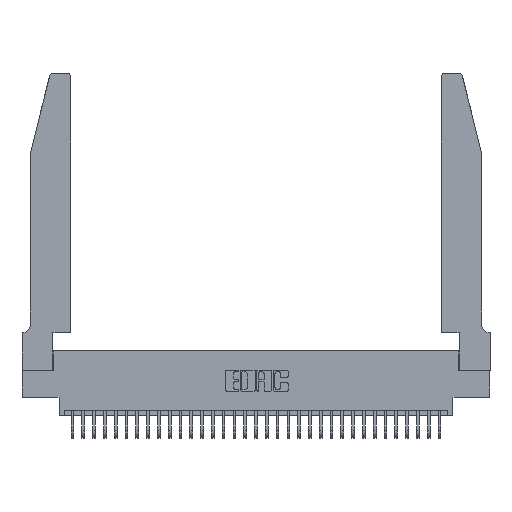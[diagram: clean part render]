
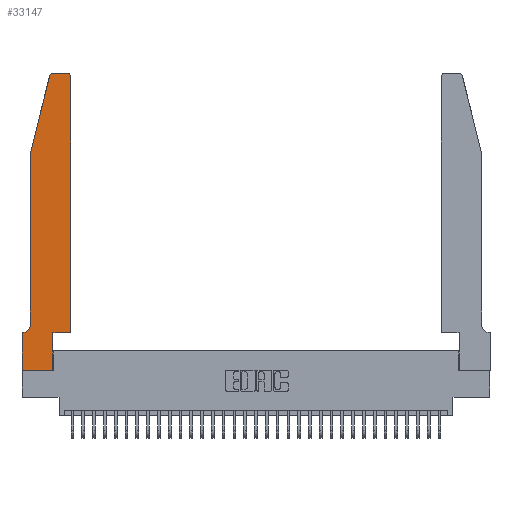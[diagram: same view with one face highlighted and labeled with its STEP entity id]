
A CAD part, top view. The second image highlights one B-rep face of the part: STEP entity #33147.
In plain terms, the highlighted planar face has unit normal (0, 0, 1).
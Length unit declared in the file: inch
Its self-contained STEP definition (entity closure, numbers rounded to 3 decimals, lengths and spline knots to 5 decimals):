
#81 = VECTOR ( 'NONE', #19132, 39.37008 ) ;
#641 = CARTESIAN_POINT ( 'NONE',  ( 0.2865, 0.35, 0.37 ) ) ;
#921 = LINE ( 'NONE', #16429, #81 ) ;
#1046 = LINE ( 'NONE', #18296, #5297 ) ;
#1325 = EDGE_CURVE ( 'NONE', #33380, #15692, #2340, .T. ) ;
#1551 = AXIS2_PLACEMENT_3D ( 'NONE', #29426, #2204, #21242 ) ;
#2133 = LINE ( 'NONE', #12270, #30064 ) ;
#2204 = DIRECTION ( 'NONE',  ( 0., 0., 1. ) ) ;
#2340 = CIRCLE ( 'NONE', #6354, 0.07 ) ;
#2687 = EDGE_LOOP ( 'NONE', ( #6096, #9109, #33235, #9890, #5475, #23231, #8841, #26085, #34514, #3562, #22490, #9394 ) ) ;
#3004 = EDGE_CURVE ( 'NONE', #22376, #18172, #30586, .T. ) ;
#3489 = CARTESIAN_POINT ( 'NONE',  ( 0.25487, 2.72718, 0.37 ) ) ;
#3562 = ORIENTED_EDGE ( 'NONE', *, *, #34745, .T. ) ;
#3617 = EDGE_CURVE ( 'NONE', #4732, #15145, #4727, .T. ) ;
#4388 = LINE ( 'NONE', #11160, #28938 ) ;
#4727 = LINE ( 'NONE', #26970, #11080 ) ;
#4732 = VERTEX_POINT ( 'NONE', #11451 ) ;
#5297 = VECTOR ( 'NONE', #26371, 39.37008 ) ;
#5475 = ORIENTED_EDGE ( 'NONE', *, *, #1325, .T. ) ;
#5584 = CARTESIAN_POINT ( 'NONE',  ( 0., 0., 0.37 ) ) ;
#6096 = ORIENTED_EDGE ( 'NONE', *, *, #33855, .T. ) ;
#6232 = CARTESIAN_POINT ( 'NONE',  ( 0.4505, 0.35, 0.37 ) ) ;
#6354 = AXIS2_PLACEMENT_3D ( 'NONE', #14543, #17375, #22728 ) ;
#7540 = CIRCLE ( 'NONE', #28967, 0.03 ) ;
#8121 = EDGE_CURVE ( 'NONE', #15692, #24479, #921, .T. ) ;
#8638 = VECTOR ( 'NONE', #23850, 39.37008 ) ;
#8841 = ORIENTED_EDGE ( 'NONE', *, *, #15777, .T. ) ;
#9016 = DIRECTION ( 'NONE',  ( 0., 0., 1. ) ) ;
#9109 = ORIENTED_EDGE ( 'NONE', *, *, #32810, .T. ) ;
#9224 = CARTESIAN_POINT ( 'NONE',  ( 0.4205, 2.72, 0.37 ) ) ;
#9394 = ORIENTED_EDGE ( 'NONE', *, *, #19500, .T. ) ;
#9439 = VERTEX_POINT ( 'NONE', #29065 ) ;
#9520 = LINE ( 'NONE', #29454, #8638 ) ;
#9890 = ORIENTED_EDGE ( 'NONE', *, *, #21620, .T. ) ;
#10090 = CARTESIAN_POINT ( 'NONE',  ( 0.4505, 2.72, 0.37 ) ) ;
#11080 = VECTOR ( 'NONE', #19087, 39.37008 ) ;
#11160 = CARTESIAN_POINT ( 'NONE',  ( 0.0755, 2., 0.37 ) ) ;
#11451 = CARTESIAN_POINT ( 'NONE',  ( 0., 0., 0.37 ) ) ;
#11564 = VECTOR ( 'NONE', #30219, 39.37008 ) ;
#11575 = DIRECTION ( 'NONE',  ( 0., 1., 0. ) ) ;
#11954 = DIRECTION ( 'NONE',  ( 0., 0., 1. ) ) ;
#12270 = CARTESIAN_POINT ( 'NONE',  ( 0.4505, 0.35, 0.37 ) ) ;
#13005 = VERTEX_POINT ( 'NONE', #14455 ) ;
#13828 = CARTESIAN_POINT ( 'NONE',  ( 0.4205, 2.75, 0.37 ) ) ;
#14339 = DIRECTION ( 'NONE',  ( 1., 0., 0. ) ) ;
#14455 = CARTESIAN_POINT ( 'NONE',  ( 0.284, 2.75, 0.37 ) ) ;
#14543 = CARTESIAN_POINT ( 'NONE',  ( 0.0055, 0.42, 0.37 ) ) ;
#14791 = DIRECTION ( 'NONE',  ( 1., 0., 0. ) ) ;
#14827 = CARTESIAN_POINT ( 'NONE',  ( 0.284, 2.72, 0.37 ) ) ;
#15145 = VERTEX_POINT ( 'NONE', #25852 ) ;
#15692 = VERTEX_POINT ( 'NONE', #34358 ) ;
#15777 = EDGE_CURVE ( 'NONE', #24479, #4732, #33645, .T. ) ;
#16429 = CARTESIAN_POINT ( 'NONE',  ( 0.0755, 0.35, 0.37 ) ) ;
#17375 = DIRECTION ( 'NONE',  ( 0., 0., -1. ) ) ;
#17505 = CARTESIAN_POINT ( 'NONE',  ( 0., 0.35, 0.37 ) ) ;
#18055 = LINE ( 'NONE', #641, #28146 ) ;
#18172 = VERTEX_POINT ( 'NONE', #27603 ) ;
#18296 = CARTESIAN_POINT ( 'NONE',  ( 0.2605, 2.75, 0.37 ) ) ;
#19087 = DIRECTION ( 'NONE',  ( 1., 0., 0. ) ) ;
#19132 = DIRECTION ( 'NONE',  ( -1., 0., 0. ) ) ;
#19500 = EDGE_CURVE ( 'NONE', #30565, #33425, #7540, .T. ) ;
#20156 = FACE_OUTER_BOUND ( 'NONE', #2687, .T. ) ;
#21242 = DIRECTION ( 'NONE',  ( 1., 0., 0. ) ) ;
#21620 = EDGE_CURVE ( 'NONE', #18172, #33380, #4388, .T. ) ;
#22376 = VERTEX_POINT ( 'NONE', #3489 ) ;
#22490 = ORIENTED_EDGE ( 'NONE', *, *, #23319, .T. ) ;
#22609 = VECTOR ( 'NONE', #30679, 39.37008 ) ;
#22728 = DIRECTION ( 'NONE',  ( -1., 0., 0. ) ) ;
#23231 = ORIENTED_EDGE ( 'NONE', *, *, #8121, .T. ) ;
#23319 = EDGE_CURVE ( 'NONE', #33542, #30565, #2133, .T. ) ;
#23587 = PLANE ( 'NONE',  #1551 ) ;
#23850 = DIRECTION ( 'NONE',  ( 1., 0., 0. ) ) ;
#24479 = VERTEX_POINT ( 'NONE', #17505 ) ;
#25852 = CARTESIAN_POINT ( 'NONE',  ( 0.2865, 0., 0.37 ) ) ;
#26085 = ORIENTED_EDGE ( 'NONE', *, *, #3617, .T. ) ;
#26371 = DIRECTION ( 'NONE',  ( -1., 0., 0. ) ) ;
#26970 = CARTESIAN_POINT ( 'NONE',  ( 0., 0., 0.37 ) ) ;
#27180 = DIRECTION ( 'NONE',  ( 0., -1., 0. ) ) ;
#27603 = CARTESIAN_POINT ( 'NONE',  ( 0.0755, 2., 0.37 ) ) ;
#28146 = VECTOR ( 'NONE', #11575, 39.37008 ) ;
#28938 = VECTOR ( 'NONE', #27180, 39.37008 ) ;
#28967 = AXIS2_PLACEMENT_3D ( 'NONE', #9224, #11954, #14791 ) ;
#29065 = CARTESIAN_POINT ( 'NONE',  ( 0.2865, 0.35, 0.37 ) ) ;
#29426 = CARTESIAN_POINT ( 'NONE',  ( 0., 0.35, 0.37 ) ) ;
#29454 = CARTESIAN_POINT ( 'NONE',  ( 0.4505, 0.35, 0.37 ) ) ;
#30064 = VECTOR ( 'NONE', #33944, 39.37008 ) ;
#30219 = DIRECTION ( 'NONE',  ( -0.239, -0.971, 0. ) ) ;
#30565 = VERTEX_POINT ( 'NONE', #10090 ) ;
#30586 = LINE ( 'NONE', #32169, #11564 ) ;
#30679 = DIRECTION ( 'NONE',  ( 0., -1., 0. ) ) ;
#32169 = CARTESIAN_POINT ( 'NONE',  ( 0.0755, 2., 0.37 ) ) ;
#32396 = CIRCLE ( 'NONE', #33024, 0.03 ) ;
#32598 = CARTESIAN_POINT ( 'NONE',  ( 0.0755, 0.42, 0.37 ) ) ;
#32810 = EDGE_CURVE ( 'NONE', #13005, #22376, #32396, .T. ) ;
#33024 = AXIS2_PLACEMENT_3D ( 'NONE', #14827, #9016, #14339 ) ;
#33147 = ADVANCED_FACE ( 'NONE', ( #20156 ), #23587, .T. ) ;
#33235 = ORIENTED_EDGE ( 'NONE', *, *, #3004, .T. ) ;
#33380 = VERTEX_POINT ( 'NONE', #32598 ) ;
#33425 = VERTEX_POINT ( 'NONE', #13828 ) ;
#33433 = EDGE_CURVE ( 'NONE', #15145, #9439, #18055, .T. ) ;
#33542 = VERTEX_POINT ( 'NONE', #6232 ) ;
#33645 = LINE ( 'NONE', #5584, #22609 ) ;
#33855 = EDGE_CURVE ( 'NONE', #33425, #13005, #1046, .T. ) ;
#33944 = DIRECTION ( 'NONE',  ( 0., 1., 0. ) ) ;
#34358 = CARTESIAN_POINT ( 'NONE',  ( 0.0055, 0.35, 0.37 ) ) ;
#34514 = ORIENTED_EDGE ( 'NONE', *, *, #33433, .T. ) ;
#34745 = EDGE_CURVE ( 'NONE', #9439, #33542, #9520, .T. ) ;
